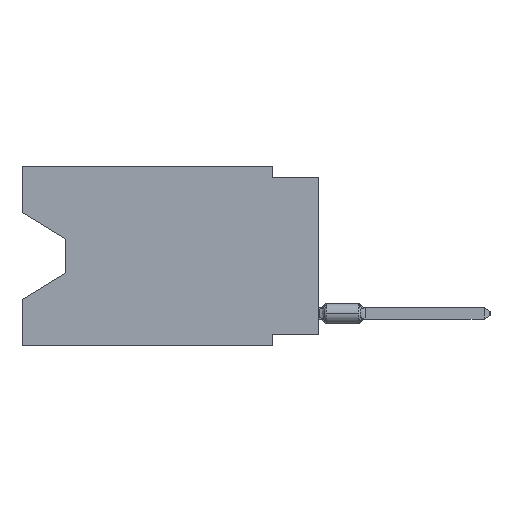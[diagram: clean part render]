
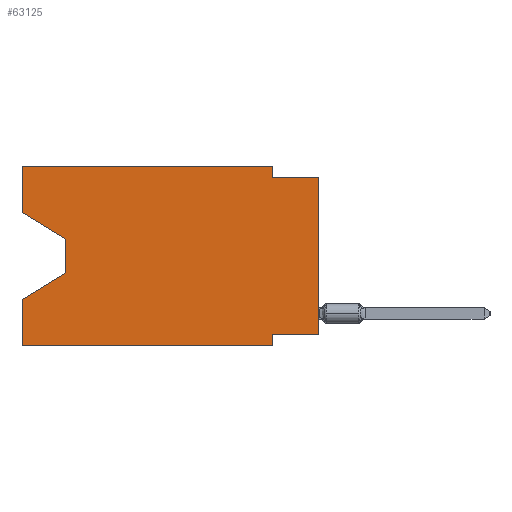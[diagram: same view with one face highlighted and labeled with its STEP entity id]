
A CAD part, left-side view. The second image highlights one B-rep face of the part: STEP entity #63125.
In plain terms, the highlighted planar face has unit normal (-1, 0, 0).
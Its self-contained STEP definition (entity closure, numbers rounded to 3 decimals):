
#558 = DIRECTION ( 'NONE',  ( 0., 0., 1. ) ) ;
#616 = CARTESIAN_POINT ( 'NONE',  ( 0., 0., 0. ) ) ;
#3188 = FACE_OUTER_BOUND ( 'NONE', #8016, .T. ) ;
#3966 = PLANE ( 'NONE',  #26159 ) ;
#4296 = VERTEX_POINT ( 'NONE', #78462 ) ;
#5063 = ORIENTED_EDGE ( 'NONE', *, *, #64582, .F. ) ;
#5623 = EDGE_CURVE ( 'NONE', #32128, #73869, #75186, .T. ) ;
#5786 = LINE ( 'NONE', #616, #63752 ) ;
#5832 = DIRECTION ( 'NONE',  ( 0., 0.855, -0.519 ) ) ;
#5910 = CARTESIAN_POINT ( 'NONE',  ( 0., 2.54, -9.271 ) ) ;
#7221 = VERTEX_POINT ( 'NONE', #31445 ) ;
#7295 = DIRECTION ( 'NONE',  ( 0., 0., -1. ) ) ;
#8016 = EDGE_LOOP ( 'NONE', ( #19088, #12720, #38117, #51199, #37558, #48794, #20788, #26268, #41840, #5063, #56974, #68333 ) ) ;
#8070 = DIRECTION ( 'NONE',  ( 0., -1., 0. ) ) ;
#9375 = CARTESIAN_POINT ( 'NONE',  ( 0., 16.383, -2.546 ) ) ;
#9649 = CARTESIAN_POINT ( 'NONE',  ( 0., 2.54, 0. ) ) ;
#9922 = DIRECTION ( 'NONE',  ( 0., 0., -1. ) ) ;
#11820 = DIRECTION ( 'NONE',  ( 0., 0., -1. ) ) ;
#12720 = ORIENTED_EDGE ( 'NONE', *, *, #38006, .T. ) ;
#13073 = CARTESIAN_POINT ( 'NONE',  ( 0., 16.383, -7.36 ) ) ;
#13533 = CARTESIAN_POINT ( 'NONE',  ( 0., 0., -0.635 ) ) ;
#14289 = VECTOR ( 'NONE', #11820, 1000. ) ;
#16444 = LINE ( 'NONE', #71677, #49792 ) ;
#16605 = EDGE_CURVE ( 'NONE', #24396, #22936, #18388, .T. ) ;
#17881 = VECTOR ( 'NONE', #60518, 1000. ) ;
#18388 = LINE ( 'NONE', #24344, #17881 ) ;
#18719 = VECTOR ( 'NONE', #558, 1000. ) ;
#19088 = ORIENTED_EDGE ( 'NONE', *, *, #77900, .T. ) ;
#20788 = ORIENTED_EDGE ( 'NONE', *, *, #58810, .F. ) ;
#22936 = VERTEX_POINT ( 'NONE', #9649 ) ;
#24344 = CARTESIAN_POINT ( 'NONE',  ( 0., 16.383, 0. ) ) ;
#24396 = VERTEX_POINT ( 'NONE', #28794 ) ;
#26159 = AXIS2_PLACEMENT_3D ( 'NONE', #46861, #34151, #9922 ) ;
#26268 = ORIENTED_EDGE ( 'NONE', *, *, #45409, .T. ) ;
#26384 = VERTEX_POINT ( 'NONE', #75958 ) ;
#27062 = LINE ( 'NONE', #52904, #75341 ) ;
#27678 = VECTOR ( 'NONE', #63417, 1000. ) ;
#28100 = VERTEX_POINT ( 'NONE', #55171 ) ;
#28794 = CARTESIAN_POINT ( 'NONE',  ( 0., 16.383, 0. ) ) ;
#29876 = EDGE_CURVE ( 'NONE', #28100, #24396, #73030, .T. ) ;
#29990 = DIRECTION ( 'NONE',  ( 0., 0., 1. ) ) ;
#30128 = VECTOR ( 'NONE', #7295, 1000. ) ;
#31445 = CARTESIAN_POINT ( 'NONE',  ( 0., 16.383, -9.906 ) ) ;
#31779 = EDGE_CURVE ( 'NONE', #7221, #41300, #61730, .T. ) ;
#32128 = VERTEX_POINT ( 'NONE', #42957 ) ;
#32253 = CARTESIAN_POINT ( 'NONE',  ( 0., 0., -9.271 ) ) ;
#34151 = DIRECTION ( 'NONE',  ( 1., 0., 0. ) ) ;
#37233 = CARTESIAN_POINT ( 'NONE',  ( 0., 13.97, -4.013 ) ) ;
#37558 = ORIENTED_EDGE ( 'NONE', *, *, #60330, .T. ) ;
#38006 = EDGE_CURVE ( 'NONE', #41150, #68290, #43219, .T. ) ;
#38117 = ORIENTED_EDGE ( 'NONE', *, *, #62459, .T. ) ;
#41150 = VERTEX_POINT ( 'NONE', #59997 ) ;
#41300 = VERTEX_POINT ( 'NONE', #13073 ) ;
#41840 = ORIENTED_EDGE ( 'NONE', *, *, #5623, .F. ) ;
#42957 = CARTESIAN_POINT ( 'NONE',  ( 0., 2.54, -0.635 ) ) ;
#43219 = LINE ( 'NONE', #37233, #14289 ) ;
#43232 = CARTESIAN_POINT ( 'NONE',  ( 0., 16.383, 0. ) ) ;
#45409 = EDGE_CURVE ( 'NONE', #26384, #73869, #5786, .T. ) ;
#46861 = CARTESIAN_POINT ( 'NONE',  ( 0., 16.383, 0. ) ) ;
#47036 = DIRECTION ( 'NONE',  ( 0., 0., -1. ) ) ;
#48230 = CARTESIAN_POINT ( 'NONE',  ( 0., 16.383, 0. ) ) ;
#48794 = ORIENTED_EDGE ( 'NONE', *, *, #67122, .F. ) ;
#49792 = VECTOR ( 'NONE', #47036, 1000. ) ;
#50216 = CARTESIAN_POINT ( 'NONE',  ( 0., 13.97, -5.893 ) ) ;
#50369 = VECTOR ( 'NONE', #61508, 1000. ) ;
#51199 = ORIENTED_EDGE ( 'NONE', *, *, #31779, .F. ) ;
#52904 = CARTESIAN_POINT ( 'NONE',  ( 0., 16.383, -9.906 ) ) ;
#55171 = CARTESIAN_POINT ( 'NONE',  ( 0., 16.383, -2.546 ) ) ;
#55782 = CARTESIAN_POINT ( 'NONE',  ( 0., 0., -0.635 ) ) ;
#56513 = DIRECTION ( 'NONE',  ( 0., 1., 0. ) ) ;
#56599 = VECTOR ( 'NONE', #5832, 1000. ) ;
#56974 = ORIENTED_EDGE ( 'NONE', *, *, #16605, .F. ) ;
#58810 = EDGE_CURVE ( 'NONE', #26384, #72658, #62466, .T. ) ;
#59997 = CARTESIAN_POINT ( 'NONE',  ( 0., 13.97, -4.013 ) ) ;
#60330 = EDGE_CURVE ( 'NONE', #7221, #4296, #27062, .T. ) ;
#60518 = DIRECTION ( 'NONE',  ( 0., -1., 0. ) ) ;
#60940 = CARTESIAN_POINT ( 'NONE',  ( 0., 2.54, 0. ) ) ;
#61508 = DIRECTION ( 'NONE',  ( 0., 0., 1. ) ) ;
#61730 = LINE ( 'NONE', #48230, #18719 ) ;
#61825 = VECTOR ( 'NONE', #8070, 1000. ) ;
#62459 = EDGE_CURVE ( 'NONE', #68290, #41300, #65434, .T. ) ;
#62466 = LINE ( 'NONE', #32253, #70097 ) ;
#63125 = ADVANCED_FACE ( 'NONE', ( #3188 ), #3966, .F. ) ;
#63417 = DIRECTION ( 'NONE',  ( 0., -0.855, -0.519 ) ) ;
#63649 = DIRECTION ( 'NONE',  ( 0., -1., 0. ) ) ;
#63752 = VECTOR ( 'NONE', #29990, 1000. ) ;
#64582 = EDGE_CURVE ( 'NONE', #22936, #32128, #73252, .T. ) ;
#65029 = CARTESIAN_POINT ( 'NONE',  ( 0., 13.97, -5.893 ) ) ;
#65434 = LINE ( 'NONE', #65029, #56599 ) ;
#67122 = EDGE_CURVE ( 'NONE', #72658, #4296, #16444, .T. ) ;
#68290 = VERTEX_POINT ( 'NONE', #50216 ) ;
#68333 = ORIENTED_EDGE ( 'NONE', *, *, #29876, .F. ) ;
#70097 = VECTOR ( 'NONE', #56513, 1000. ) ;
#71677 = CARTESIAN_POINT ( 'NONE',  ( 0., 2.54, -9.906 ) ) ;
#72658 = VERTEX_POINT ( 'NONE', #5910 ) ;
#73030 = LINE ( 'NONE', #43232, #50369 ) ;
#73252 = LINE ( 'NONE', #60940, #30128 ) ;
#73869 = VERTEX_POINT ( 'NONE', #13533 ) ;
#74266 = LINE ( 'NONE', #9375, #27678 ) ;
#75186 = LINE ( 'NONE', #55782, #61825 ) ;
#75341 = VECTOR ( 'NONE', #63649, 1000. ) ;
#75958 = CARTESIAN_POINT ( 'NONE',  ( 0., 0., -9.271 ) ) ;
#77900 = EDGE_CURVE ( 'NONE', #28100, #41150, #74266, .T. ) ;
#78462 = CARTESIAN_POINT ( 'NONE',  ( 0., 2.54, -9.906 ) ) ;
